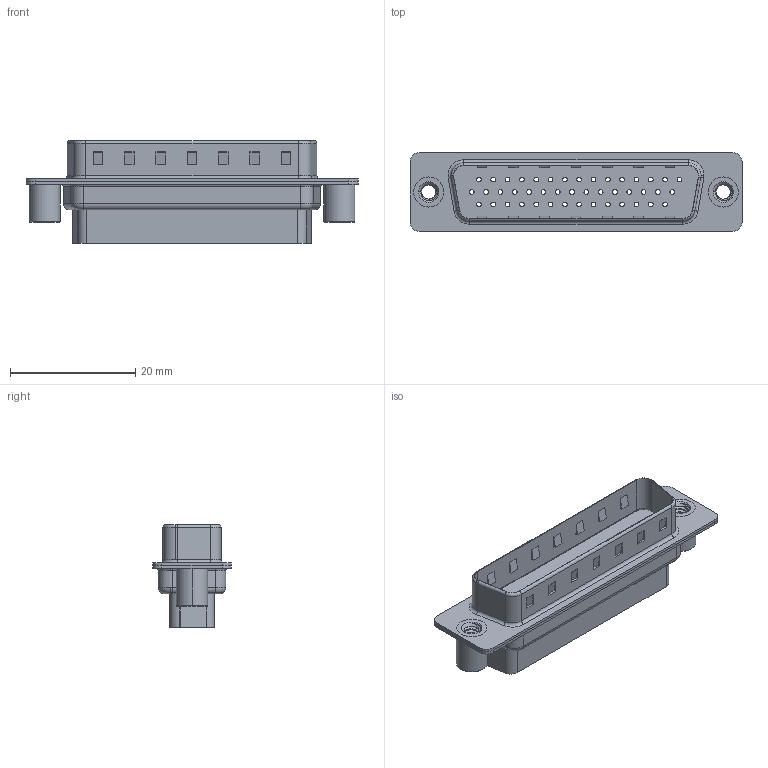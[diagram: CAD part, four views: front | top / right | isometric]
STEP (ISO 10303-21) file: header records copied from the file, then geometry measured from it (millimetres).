
FILE_DESCRIPTION (( 'STEP AP203' ), '1' );
FILE_NAME ('637-044-010-249.STEP', '2020-07-17T21:24:09', ( '' ), ( '' ), 'SwSTEP 2.0', 'SolidWorks 2020', '' );
FILE_SCHEMA (( 'CONFIG_CONTROL_DESIGN' ));
Length unit declared in the file: millimetre
Products named in the file (5): 637 Shell Rear_44 Contacts; 637 Housing_44 Contacts HP; 637 4-40 Threaded Standoff BS; 637 Shell Front_44 Contacts; 637-044-010-249
Assembly tree (5 placements, depth 2):
  637-044-010-249
    637 Housing_44 Contacts HP
    637 Shell Front_44 Contacts
    637 Shell Rear_44 Contacts
    637 4-40 Threaded Standoff BS  x2
Bounding box: 53 x 12.6 x 16.4 mm (x, y, z)
Volume: 3074.2 mm3; surface area: 7517.5 mm2
Topology: 5 solids, 5 shells, 750 faces, 1813 edges, 1172 vertices
Faces by surface type: cylinder 421, plane 259, torus 50, cone 14, bspline 6
Entity records: 23193 total; most frequent: CARTESIAN_POINT 5300, DIRECTION 3873, ORIENTED_EDGE 3400, EDGE_CURVE 1700, AXIS2_PLACEMENT_3D 1529, VERTEX_POINT 1099, EDGE_LOOP 933, CIRCLE 818
